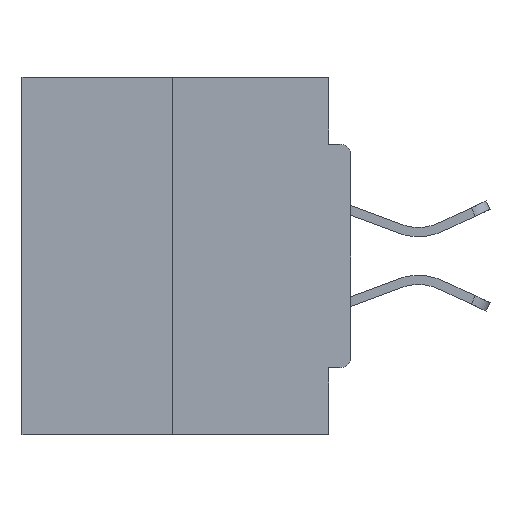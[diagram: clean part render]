
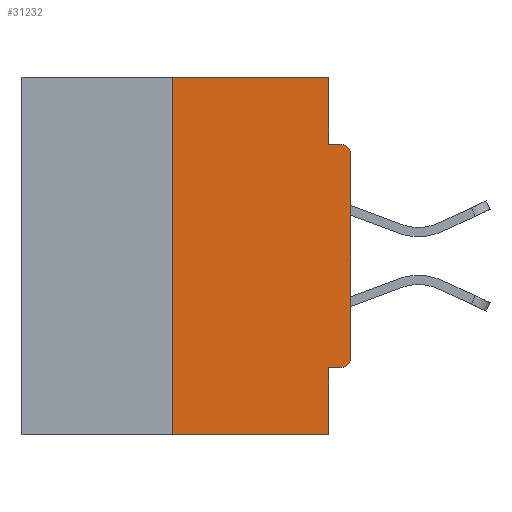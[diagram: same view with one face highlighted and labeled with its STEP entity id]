
A CAD part, left-side view. The second image highlights one B-rep face of the part: STEP entity #31232.
In plain terms, the highlighted planar face has unit normal (-1, 0, 0).
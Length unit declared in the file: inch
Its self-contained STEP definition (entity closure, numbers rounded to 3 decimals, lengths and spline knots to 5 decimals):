
#288 = CARTESIAN_POINT ( 'NONE',  ( 0., 0.46, 0. ) ) ;
#794 = VERTEX_POINT ( 'NONE', #905 ) ;
#884 = VERTEX_POINT ( 'NONE', #27418 ) ;
#905 = CARTESIAN_POINT ( 'NONE',  ( 0., 0.25, -0.5 ) ) ;
#1160 = LINE ( 'NONE', #6723, #31862 ) ;
#1469 = ORIENTED_EDGE ( 'NONE', *, *, #5833, .T. ) ;
#1493 = LINE ( 'NONE', #24818, #30414 ) ;
#1853 = LINE ( 'NONE', #33781, #29870 ) ;
#3076 = CARTESIAN_POINT ( 'NONE',  ( 0., 0., -0.3915 ) ) ;
#3129 = CARTESIAN_POINT ( 'NONE',  ( 0., 0.015, -0.4065 ) ) ;
#3210 = ORIENTED_EDGE ( 'NONE', *, *, #18881, .F. ) ;
#3629 = ORIENTED_EDGE ( 'NONE', *, *, #28941, .F. ) ;
#4288 = EDGE_CURVE ( 'NONE', #21265, #884, #32841, .T. ) ;
#4615 = AXIS2_PLACEMENT_3D ( 'NONE', #21883, #13264, #4824 ) ;
#4824 = DIRECTION ( 'NONE',  ( 0., 0., -1. ) ) ;
#5048 = LINE ( 'NONE', #23500, #8199 ) ;
#5149 = CARTESIAN_POINT ( 'NONE',  ( 0., 0.031, -0.4065 ) ) ;
#5833 = EDGE_CURVE ( 'NONE', #30318, #33177, #19180, .T. ) ;
#5902 = CIRCLE ( 'NONE', #4615, 0.015 ) ;
#5927 = CARTESIAN_POINT ( 'NONE',  ( 0., 0., -0.1085 ) ) ;
#6723 = CARTESIAN_POINT ( 'NONE',  ( 0., 0.031, 0. ) ) ;
#7153 = DIRECTION ( 'NONE',  ( 0., -1., 0. ) ) ;
#8199 = VECTOR ( 'NONE', #14605, 39.37008 ) ;
#8692 = EDGE_CURVE ( 'NONE', #32268, #10284, #5902, .T. ) ;
#9873 = VERTEX_POINT ( 'NONE', #5149 ) ;
#10284 = VERTEX_POINT ( 'NONE', #3076 ) ;
#11226 = EDGE_CURVE ( 'NONE', #9873, #29394, #1853, .T. ) ;
#13264 = DIRECTION ( 'NONE',  ( -1., 0., 0. ) ) ;
#13368 = VECTOR ( 'NONE', #26585, 39.37008 ) ;
#14314 = CARTESIAN_POINT ( 'NONE',  ( 0., 0.25, 0. ) ) ;
#14605 = DIRECTION ( 'NONE',  ( 0., 0., 1. ) ) ;
#15646 = ORIENTED_EDGE ( 'NONE', *, *, #20986, .F. ) ;
#16116 = EDGE_CURVE ( 'NONE', #794, #29394, #1493, .T. ) ;
#17322 = DIRECTION ( 'NONE',  ( 0., 1., 0. ) ) ;
#17830 = DIRECTION ( 'NONE',  ( 0., -1., 0. ) ) ;
#18040 = CARTESIAN_POINT ( 'NONE',  ( 0., 0.031, -0.5 ) ) ;
#18749 = DIRECTION ( 'NONE',  ( 1., 0., 0. ) ) ;
#18752 = ORIENTED_EDGE ( 'NONE', *, *, #24819, .T. ) ;
#18881 = EDGE_CURVE ( 'NONE', #32268, #9873, #22431, .T. ) ;
#19180 = CIRCLE ( 'NONE', #32217, 0.015 ) ;
#19281 = DIRECTION ( 'NONE',  ( 0., 0., -1. ) ) ;
#20223 = AXIS2_PLACEMENT_3D ( 'NONE', #29872, #18749, #24333 ) ;
#20854 = CARTESIAN_POINT ( 'NONE',  ( 0., 0.25, 0. ) ) ;
#20881 = CARTESIAN_POINT ( 'NONE',  ( 0., 0., -0.0935 ) ) ;
#20986 = EDGE_CURVE ( 'NONE', #794, #21265, #34436, .T. ) ;
#21265 = VERTEX_POINT ( 'NONE', #14314 ) ;
#21883 = CARTESIAN_POINT ( 'NONE',  ( 0., 0.015, -0.3915 ) ) ;
#22186 = DIRECTION ( 'NONE',  ( -1., 0., 0. ) ) ;
#22320 = ORIENTED_EDGE ( 'NONE', *, *, #31986, .F. ) ;
#22431 = LINE ( 'NONE', #25610, #26963 ) ;
#22443 = ORIENTED_EDGE ( 'NONE', *, *, #11226, .F. ) ;
#23500 = CARTESIAN_POINT ( 'NONE',  ( 0., 0., 0. ) ) ;
#23650 = DIRECTION ( 'NONE',  ( 0., 0., 1. ) ) ;
#23904 = DIRECTION ( 'NONE',  ( 0., 0., -1. ) ) ;
#24285 = CARTESIAN_POINT ( 'NONE',  ( 0., 0.015, -0.0935 ) ) ;
#24333 = DIRECTION ( 'NONE',  ( 0., 0., -1. ) ) ;
#24614 = VERTEX_POINT ( 'NONE', #30703 ) ;
#24818 = CARTESIAN_POINT ( 'NONE',  ( 0., 0.46, -0.5 ) ) ;
#24819 = EDGE_CURVE ( 'NONE', #10284, #30318, #5048, .T. ) ;
#24988 = CARTESIAN_POINT ( 'NONE',  ( 0., 0.015, -0.1085 ) ) ;
#25584 = EDGE_LOOP ( 'NONE', ( #26577, #15646, #34499, #22443, #3210, #36095, #18752, #1469, #3629, #22320 ) ) ;
#25610 = CARTESIAN_POINT ( 'NONE',  ( 0., 0., -0.4065 ) ) ;
#25642 = VECTOR ( 'NONE', #17830, 39.37008 ) ;
#26328 = VECTOR ( 'NONE', #23650, 39.37008 ) ;
#26573 = FACE_OUTER_BOUND ( 'NONE', #25584, .T. ) ;
#26577 = ORIENTED_EDGE ( 'NONE', *, *, #4288, .F. ) ;
#26585 = DIRECTION ( 'NONE',  ( 0., -1., 0. ) ) ;
#26963 = VECTOR ( 'NONE', #17322, 39.37008 ) ;
#27418 = CARTESIAN_POINT ( 'NONE',  ( 0., 0.031, 0. ) ) ;
#27476 = PLANE ( 'NONE',  #20223 ) ;
#28104 = DIRECTION ( 'NONE',  ( 0., 0., -1. ) ) ;
#28941 = EDGE_CURVE ( 'NONE', #24614, #33177, #34421, .T. ) ;
#29394 = VERTEX_POINT ( 'NONE', #18040 ) ;
#29870 = VECTOR ( 'NONE', #28104, 39.37008 ) ;
#29872 = CARTESIAN_POINT ( 'NONE',  ( 0., 0.46, 0. ) ) ;
#30318 = VERTEX_POINT ( 'NONE', #5927 ) ;
#30414 = VECTOR ( 'NONE', #7153, 39.37008 ) ;
#30703 = CARTESIAN_POINT ( 'NONE',  ( 0., 0.031, -0.0935 ) ) ;
#31232 = ADVANCED_FACE ( 'NONE', ( #26573 ), #27476, .F. ) ;
#31862 = VECTOR ( 'NONE', #23904, 39.37008 ) ;
#31986 = EDGE_CURVE ( 'NONE', #884, #24614, #1160, .T. ) ;
#32217 = AXIS2_PLACEMENT_3D ( 'NONE', #24988, #22186, #19281 ) ;
#32268 = VERTEX_POINT ( 'NONE', #3129 ) ;
#32841 = LINE ( 'NONE', #288, #13368 ) ;
#33177 = VERTEX_POINT ( 'NONE', #24285 ) ;
#33781 = CARTESIAN_POINT ( 'NONE',  ( 0., 0.031, -0.5 ) ) ;
#34421 = LINE ( 'NONE', #20881, #25642 ) ;
#34436 = LINE ( 'NONE', #20854, #26328 ) ;
#34499 = ORIENTED_EDGE ( 'NONE', *, *, #16116, .T. ) ;
#36095 = ORIENTED_EDGE ( 'NONE', *, *, #8692, .T. ) ;
